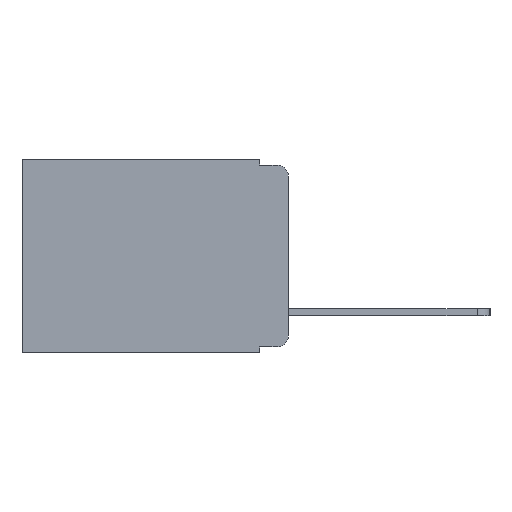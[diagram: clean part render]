
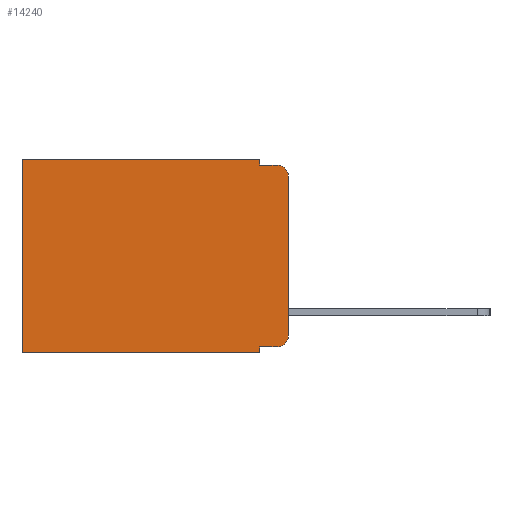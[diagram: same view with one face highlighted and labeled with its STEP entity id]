
A CAD part, left-side view. The second image highlights one B-rep face of the part: STEP entity #14240.
In plain terms, the highlighted planar face has unit normal (-1, 0, 0).
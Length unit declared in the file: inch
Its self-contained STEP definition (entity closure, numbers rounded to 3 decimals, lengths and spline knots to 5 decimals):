
#65 = EDGE_CURVE ( 'NONE', #4712, #10384, #16435, .T. ) ;
#520 = ORIENTED_EDGE ( 'NONE', *, *, #2689, .F. ) ;
#632 = VECTOR ( 'NONE', #20532, 39.37008 ) ;
#1102 = CARTESIAN_POINT ( 'NONE',  ( 0.298, 0.051, 0. ) ) ;
#1613 = PLANE ( 'NONE',  #23206 ) ;
#1738 = CARTESIAN_POINT ( 'NONE',  ( 0.298, 0.02, -0.01 ) ) ;
#1857 = EDGE_CURVE ( 'NONE', #11543, #18144, #5669, .T. ) ;
#1958 = DIRECTION ( 'NONE',  ( -1., 0., 0. ) ) ;
#2689 = EDGE_CURVE ( 'NONE', #9902, #4782, #11322, .T. ) ;
#2810 = CARTESIAN_POINT ( 'NONE',  ( 0.298, 0., -0.313 ) ) ;
#2903 = VECTOR ( 'NONE', #22986, 39.37008 ) ;
#2912 = EDGE_LOOP ( 'NONE', ( #5646, #21334, #8316, #8284, #11727, #5593, #24130, #520, #20452, #6466 ) ) ;
#3188 = FACE_OUTER_BOUND ( 'NONE', #2912, .T. ) ;
#3754 = VECTOR ( 'NONE', #17222, 39.37008 ) ;
#4165 = VECTOR ( 'NONE', #5208, 39.37008 ) ;
#4380 = CARTESIAN_POINT ( 'NONE',  ( 0.298, 0.473, 0. ) ) ;
#4712 = VERTEX_POINT ( 'NONE', #4380 ) ;
#4782 = VERTEX_POINT ( 'NONE', #5328 ) ;
#5208 = DIRECTION ( 'NONE',  ( 0., 1., 0. ) ) ;
#5328 = CARTESIAN_POINT ( 'NONE',  ( 0.298, 0.051, -0.343 ) ) ;
#5482 = DIRECTION ( 'NONE',  ( 0., 0., -1. ) ) ;
#5593 = ORIENTED_EDGE ( 'NONE', *, *, #65, .T. ) ;
#5626 = CARTESIAN_POINT ( 'NONE',  ( 0.298, 0.02, -0.333 ) ) ;
#5646 = ORIENTED_EDGE ( 'NONE', *, *, #17621, .F. ) ;
#5669 = CIRCLE ( 'NONE', #11362, 0.02 ) ;
#6466 = ORIENTED_EDGE ( 'NONE', *, *, #15412, .T. ) ;
#6878 = DIRECTION ( 'NONE',  ( 0., 0., -1. ) ) ;
#7057 = CARTESIAN_POINT ( 'NONE',  ( 0.298, 0.02, -0.313 ) ) ;
#7120 = DIRECTION ( 'NONE',  ( 0., -1., 0. ) ) ;
#7611 = CARTESIAN_POINT ( 'NONE',  ( 0.298, 0.473, -0.343 ) ) ;
#8147 = CARTESIAN_POINT ( 'NONE',  ( 0.298, 0.02, -0.03 ) ) ;
#8284 = ORIENTED_EDGE ( 'NONE', *, *, #15874, .F. ) ;
#8316 = ORIENTED_EDGE ( 'NONE', *, *, #12055, .F. ) ;
#8326 = LINE ( 'NONE', #23723, #17236 ) ;
#8736 = VERTEX_POINT ( 'NONE', #2810 ) ;
#8849 = CARTESIAN_POINT ( 'NONE',  ( 0.298, 0., -0.343 ) ) ;
#8866 = EDGE_CURVE ( 'NONE', #4782, #10384, #23754, .T. ) ;
#8971 = DIRECTION ( 'NONE',  ( 0., 0., -1. ) ) ;
#9184 = LINE ( 'NONE', #23941, #4165 ) ;
#9359 = LINE ( 'NONE', #9660, #3754 ) ;
#9660 = CARTESIAN_POINT ( 'NONE',  ( 0.298, 0., 0. ) ) ;
#9902 = VERTEX_POINT ( 'NONE', #19885 ) ;
#10004 = LINE ( 'NONE', #14701, #14480 ) ;
#10384 = VERTEX_POINT ( 'NONE', #7611 ) ;
#11117 = CARTESIAN_POINT ( 'NONE',  ( 0.298, 0., -0.03 ) ) ;
#11251 = AXIS2_PLACEMENT_3D ( 'NONE', #7057, #20291, #8971 ) ;
#11322 = LINE ( 'NONE', #1102, #20790 ) ;
#11362 = AXIS2_PLACEMENT_3D ( 'NONE', #8147, #1958, #6878 ) ;
#11543 = VERTEX_POINT ( 'NONE', #11117 ) ;
#11727 = ORIENTED_EDGE ( 'NONE', *, *, #12626, .T. ) ;
#11843 = CARTESIAN_POINT ( 'NONE',  ( 0.298, 0.051, -0.01 ) ) ;
#12055 = EDGE_CURVE ( 'NONE', #12424, #18144, #8326, .T. ) ;
#12424 = VERTEX_POINT ( 'NONE', #11843 ) ;
#12626 = EDGE_CURVE ( 'NONE', #23107, #4712, #9184, .T. ) ;
#13853 = VECTOR ( 'NONE', #18386, 39.37008 ) ;
#14167 = EDGE_CURVE ( 'NONE', #9902, #18073, #10004, .T. ) ;
#14240 = ADVANCED_FACE ( 'NONE', ( #3188 ), #1613, .F. ) ;
#14480 = VECTOR ( 'NONE', #7120, 39.37008 ) ;
#14701 = CARTESIAN_POINT ( 'NONE',  ( 0.298, 0.051, -0.333 ) ) ;
#14922 = CARTESIAN_POINT ( 'NONE',  ( 0.298, 0., 0. ) ) ;
#15412 = EDGE_CURVE ( 'NONE', #18073, #8736, #18642, .T. ) ;
#15874 = EDGE_CURVE ( 'NONE', #23107, #12424, #18032, .T. ) ;
#16435 = LINE ( 'NONE', #20555, #632 ) ;
#16828 = DIRECTION ( 'NONE',  ( 1., 0., 0. ) ) ;
#17222 = DIRECTION ( 'NONE',  ( 0., 0., -1. ) ) ;
#17236 = VECTOR ( 'NONE', #20192, 39.37008 ) ;
#17621 = EDGE_CURVE ( 'NONE', #11543, #8736, #9359, .T. ) ;
#18032 = LINE ( 'NONE', #19343, #2903 ) ;
#18073 = VERTEX_POINT ( 'NONE', #5626 ) ;
#18144 = VERTEX_POINT ( 'NONE', #1738 ) ;
#18386 = DIRECTION ( 'NONE',  ( 0., 1., 0. ) ) ;
#18609 = DIRECTION ( 'NONE',  ( 0., 0., -1. ) ) ;
#18642 = CIRCLE ( 'NONE', #11251, 0.02 ) ;
#19343 = CARTESIAN_POINT ( 'NONE',  ( 0.298, 0.051, 0. ) ) ;
#19885 = CARTESIAN_POINT ( 'NONE',  ( 0.298, 0.051, -0.333 ) ) ;
#20187 = CARTESIAN_POINT ( 'NONE',  ( 0.298, 0.051, 0. ) ) ;
#20192 = DIRECTION ( 'NONE',  ( 0., -1., 0. ) ) ;
#20291 = DIRECTION ( 'NONE',  ( -1., 0., 0. ) ) ;
#20452 = ORIENTED_EDGE ( 'NONE', *, *, #14167, .T. ) ;
#20532 = DIRECTION ( 'NONE',  ( 0., 0., -1. ) ) ;
#20555 = CARTESIAN_POINT ( 'NONE',  ( 0.298, 0.473, 0. ) ) ;
#20790 = VECTOR ( 'NONE', #18609, 39.37008 ) ;
#21334 = ORIENTED_EDGE ( 'NONE', *, *, #1857, .T. ) ;
#22986 = DIRECTION ( 'NONE',  ( 0., 0., -1. ) ) ;
#23107 = VERTEX_POINT ( 'NONE', #20187 ) ;
#23206 = AXIS2_PLACEMENT_3D ( 'NONE', #14922, #16828, #5482 ) ;
#23723 = CARTESIAN_POINT ( 'NONE',  ( 0.298, 0.051, -0.01 ) ) ;
#23754 = LINE ( 'NONE', #8849, #13853 ) ;
#23941 = CARTESIAN_POINT ( 'NONE',  ( 0.298, 0., 0. ) ) ;
#24130 = ORIENTED_EDGE ( 'NONE', *, *, #8866, .F. ) ;
